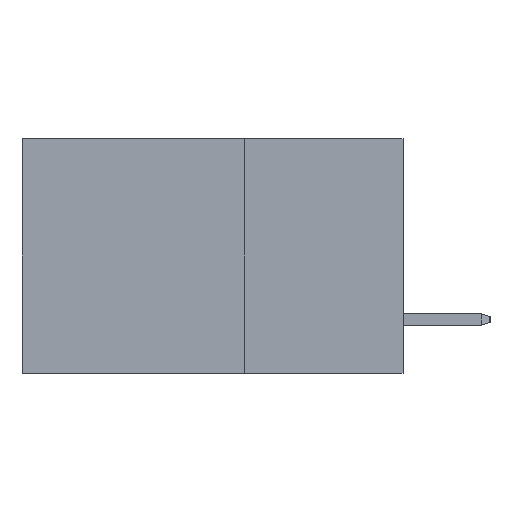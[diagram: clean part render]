
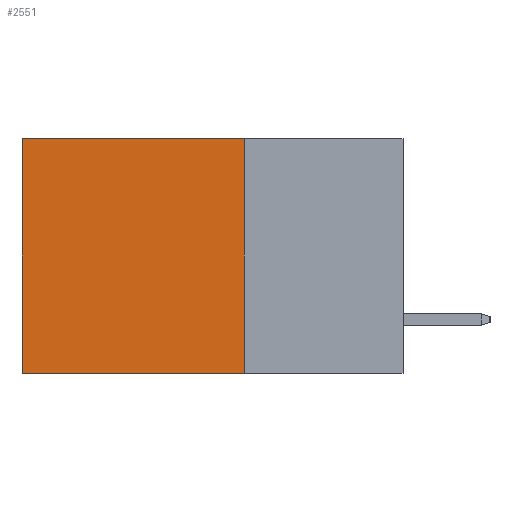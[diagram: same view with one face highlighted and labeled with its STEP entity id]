
A CAD part, left-side view. The second image highlights one B-rep face of the part: STEP entity #2551.
In plain terms, the highlighted planar face has unit normal (-1, 0, 0).
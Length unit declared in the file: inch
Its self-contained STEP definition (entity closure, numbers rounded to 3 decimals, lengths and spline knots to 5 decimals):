
#45 = PLANE ( 'NONE',  #8995 ) ;
#952 = LINE ( 'NONE', #1047, #8948 ) ;
#1025 = ORIENTED_EDGE ( 'NONE', *, *, #6970, .T. ) ;
#1047 = CARTESIAN_POINT ( 'NONE',  ( 0.2875, 0.25, 0. ) ) ;
#1343 = VECTOR ( 'NONE', #7961, 39.37008 ) ;
#1528 = LINE ( 'NONE', #7220, #4497 ) ;
#1539 = ORIENTED_EDGE ( 'NONE', *, *, #3085, .F. ) ;
#1741 = LINE ( 'NONE', #9926, #1343 ) ;
#1798 = CARTESIAN_POINT ( 'NONE',  ( 0.2875, 0.25, 0. ) ) ;
#1876 = EDGE_CURVE ( 'NONE', #2397, #6628, #8270, .T. ) ;
#2343 = CARTESIAN_POINT ( 'NONE',  ( 0.2875, 0.25, -0.37 ) ) ;
#2397 = VERTEX_POINT ( 'NONE', #6184 ) ;
#2454 = ORIENTED_EDGE ( 'NONE', *, *, #1876, .T. ) ;
#2551 = ADVANCED_FACE ( 'NONE', ( #8939 ), #45, .F. ) ;
#3085 = EDGE_CURVE ( 'NONE', #2397, #5677, #952, .T. ) ;
#3225 = DIRECTION ( 'NONE',  ( 0., 0., -1. ) ) ;
#3255 = CARTESIAN_POINT ( 'NONE',  ( 0.2875, 0.6, -0.37 ) ) ;
#3504 = VERTEX_POINT ( 'NONE', #3255 ) ;
#4497 = VECTOR ( 'NONE', #8242, 39.37008 ) ;
#4710 = VECTOR ( 'NONE', #8419, 39.37008 ) ;
#5677 = VERTEX_POINT ( 'NONE', #2343 ) ;
#6029 = EDGE_CURVE ( 'NONE', #5677, #3504, #1528, .T. ) ;
#6184 = CARTESIAN_POINT ( 'NONE',  ( 0.2875, 0.25, 0. ) ) ;
#6628 = VERTEX_POINT ( 'NONE', #9895 ) ;
#6970 = EDGE_CURVE ( 'NONE', #6628, #3504, #1741, .T. ) ;
#7160 = ORIENTED_EDGE ( 'NONE', *, *, #6029, .F. ) ;
#7175 = EDGE_LOOP ( 'NONE', ( #1025, #7160, #1539, #2454 ) ) ;
#7220 = CARTESIAN_POINT ( 'NONE',  ( 0.2875, 0.25, -0.37 ) ) ;
#7364 = CARTESIAN_POINT ( 'NONE',  ( 0.2875, 0.25, 0. ) ) ;
#7410 = DIRECTION ( 'NONE',  ( 1., 0., 0. ) ) ;
#7961 = DIRECTION ( 'NONE',  ( 0., 0., -1. ) ) ;
#8242 = DIRECTION ( 'NONE',  ( 0., 1., 0. ) ) ;
#8270 = LINE ( 'NONE', #1798, #4710 ) ;
#8419 = DIRECTION ( 'NONE',  ( 0., 1., 0. ) ) ;
#8939 = FACE_OUTER_BOUND ( 'NONE', #7175, .T. ) ;
#8948 = VECTOR ( 'NONE', #10078, 39.37008 ) ;
#8995 = AXIS2_PLACEMENT_3D ( 'NONE', #7364, #7410, #3225 ) ;
#9895 = CARTESIAN_POINT ( 'NONE',  ( 0.2875, 0.6, 0. ) ) ;
#9926 = CARTESIAN_POINT ( 'NONE',  ( 0.2875, 0.6, 0. ) ) ;
#10078 = DIRECTION ( 'NONE',  ( 0., 0., -1. ) ) ;
